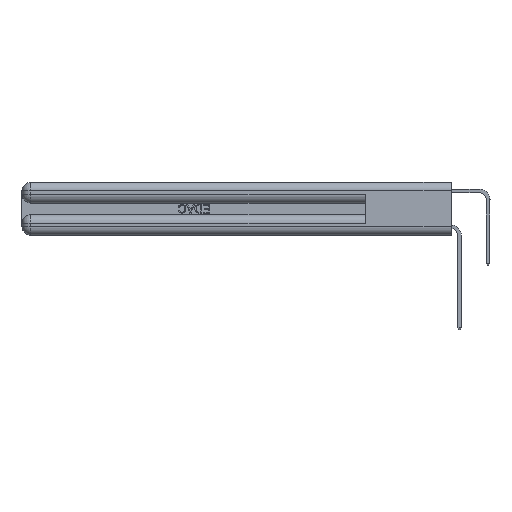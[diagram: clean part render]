
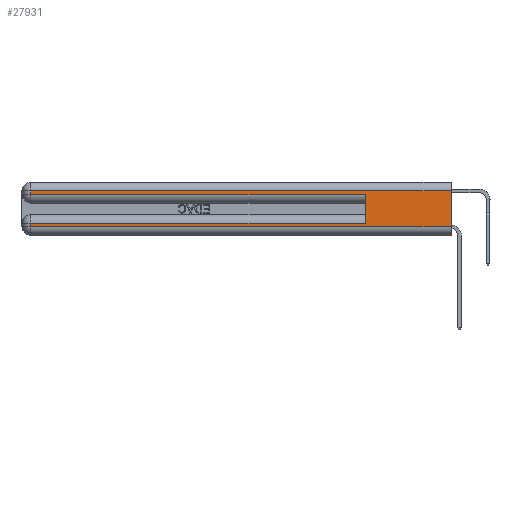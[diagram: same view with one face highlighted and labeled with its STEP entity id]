
A CAD part, left-side view. The second image highlights one B-rep face of the part: STEP entity #27931.
In plain terms, the highlighted planar face has unit normal (-1, 0, 0).
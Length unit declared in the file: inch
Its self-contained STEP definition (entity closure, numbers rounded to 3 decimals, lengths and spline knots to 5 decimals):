
#249 = LINE ( 'NONE', #35592, #9337 ) ;
#373 = DIRECTION ( 'NONE',  ( 0., 0., -1. ) ) ;
#705 = DIRECTION ( 'NONE',  ( 0., -1., 0. ) ) ;
#1419 = AXIS2_PLACEMENT_3D ( 'NONE', #9784, #21494, #373 ) ;
#1732 = VECTOR ( 'NONE', #36423, 39.37008 ) ;
#2411 = ORIENTED_EDGE ( 'NONE', *, *, #12230, .T. ) ;
#4476 = VECTOR ( 'NONE', #16833, 39.37008 ) ;
#4673 = CARTESIAN_POINT ( 'NONE',  ( 0., 0., 0.31 ) ) ;
#5842 = VERTEX_POINT ( 'NONE', #13808 ) ;
#6014 = EDGE_CURVE ( 'NONE', #24967, #21739, #35115, .T. ) ;
#6152 = VECTOR ( 'NONE', #705, 39.37008 ) ;
#6254 = EDGE_LOOP ( 'NONE', ( #32831, #10656, #37155, #32380, #8347, #20932, #2411, #20665 ) ) ;
#6481 = LINE ( 'NONE', #18212, #17121 ) ;
#6525 = FACE_OUTER_BOUND ( 'NONE', #6254, .T. ) ;
#8036 = DIRECTION ( 'NONE',  ( 0., 0., -1. ) ) ;
#8347 = ORIENTED_EDGE ( 'NONE', *, *, #10872, .F. ) ;
#8356 = EDGE_CURVE ( 'NONE', #30000, #5842, #249, .T. ) ;
#8436 = LINE ( 'NONE', #17851, #20967 ) ;
#8553 = LINE ( 'NONE', #17205, #4476 ) ;
#9337 = VECTOR ( 'NONE', #29660, 39.37008 ) ;
#9784 = CARTESIAN_POINT ( 'NONE',  ( 0., 0., 0.37 ) ) ;
#10306 = LINE ( 'NONE', #24706, #1732 ) ;
#10656 = ORIENTED_EDGE ( 'NONE', *, *, #8356, .T. ) ;
#10872 = EDGE_CURVE ( 'NONE', #27392, #21739, #24145, .T. ) ;
#10893 = VECTOR ( 'NONE', #20517, 39.37008 ) ;
#11085 = CARTESIAN_POINT ( 'NONE',  ( 0., 2.94, 0.285 ) ) ;
#11926 = VERTEX_POINT ( 'NONE', #35761 ) ;
#12055 = CARTESIAN_POINT ( 'NONE',  ( 0., 0.6, 0.145 ) ) ;
#12230 = EDGE_CURVE ( 'NONE', #20952, #15906, #6481, .T. ) ;
#13808 = CARTESIAN_POINT ( 'NONE',  ( 0., 2.94, 0.31 ) ) ;
#14168 = CARTESIAN_POINT ( 'NONE',  ( 0., 2.94, 0.37 ) ) ;
#14885 = CARTESIAN_POINT ( 'NONE',  ( 0., 0.6, 0.285 ) ) ;
#15906 = VERTEX_POINT ( 'NONE', #27173 ) ;
#16752 = EDGE_CURVE ( 'NONE', #30000, #11926, #10306, .T. ) ;
#16833 = DIRECTION ( 'NONE',  ( 0., -1., 0. ) ) ;
#17121 = VECTOR ( 'NONE', #24711, 39.37008 ) ;
#17205 = CARTESIAN_POINT ( 'NONE',  ( 0., 0., 0.06 ) ) ;
#17851 = CARTESIAN_POINT ( 'NONE',  ( 0., 0., 0.085 ) ) ;
#17974 = CARTESIAN_POINT ( 'NONE',  ( 0., 0.6, 0.085 ) ) ;
#18212 = CARTESIAN_POINT ( 'NONE',  ( 0., 2.94, 0.37 ) ) ;
#18221 = EDGE_CURVE ( 'NONE', #27392, #20952, #8436, .T. ) ;
#20167 = DIRECTION ( 'NONE',  ( 0., 1., 0. ) ) ;
#20517 = DIRECTION ( 'NONE',  ( 0., 0., 1. ) ) ;
#20665 = ORIENTED_EDGE ( 'NONE', *, *, #27240, .T. ) ;
#20932 = ORIENTED_EDGE ( 'NONE', *, *, #18221, .T. ) ;
#20952 = VERTEX_POINT ( 'NONE', #36088 ) ;
#20967 = VECTOR ( 'NONE', #20167, 39.37008 ) ;
#21281 = CARTESIAN_POINT ( 'NONE',  ( 0., 0., 0.285 ) ) ;
#21494 = DIRECTION ( 'NONE',  ( 1., 0., 0. ) ) ;
#21739 = VERTEX_POINT ( 'NONE', #14885 ) ;
#22644 = LINE ( 'NONE', #14168, #30021 ) ;
#24145 = LINE ( 'NONE', #12055, #10893 ) ;
#24706 = CARTESIAN_POINT ( 'NONE',  ( 0., 0., 0.37 ) ) ;
#24711 = DIRECTION ( 'NONE',  ( 0., 0., -1. ) ) ;
#24967 = VERTEX_POINT ( 'NONE', #11085 ) ;
#27173 = CARTESIAN_POINT ( 'NONE',  ( 0., 2.94, 0.06 ) ) ;
#27240 = EDGE_CURVE ( 'NONE', #15906, #11926, #8553, .T. ) ;
#27392 = VERTEX_POINT ( 'NONE', #17974 ) ;
#27931 = ADVANCED_FACE ( 'NONE', ( #6525 ), #29966, .F. ) ;
#28246 = EDGE_CURVE ( 'NONE', #5842, #24967, #22644, .T. ) ;
#29660 = DIRECTION ( 'NONE',  ( 0., 1., 0. ) ) ;
#29966 = PLANE ( 'NONE',  #1419 ) ;
#30000 = VERTEX_POINT ( 'NONE', #4673 ) ;
#30021 = VECTOR ( 'NONE', #8036, 39.37008 ) ;
#32380 = ORIENTED_EDGE ( 'NONE', *, *, #6014, .T. ) ;
#32831 = ORIENTED_EDGE ( 'NONE', *, *, #16752, .F. ) ;
#35115 = LINE ( 'NONE', #21281, #6152 ) ;
#35592 = CARTESIAN_POINT ( 'NONE',  ( 0., 0., 0.31 ) ) ;
#35761 = CARTESIAN_POINT ( 'NONE',  ( 0., 0., 0.06 ) ) ;
#36088 = CARTESIAN_POINT ( 'NONE',  ( 0., 2.94, 0.085 ) ) ;
#36423 = DIRECTION ( 'NONE',  ( 0., 0., -1. ) ) ;
#37155 = ORIENTED_EDGE ( 'NONE', *, *, #28246, .T. ) ;
